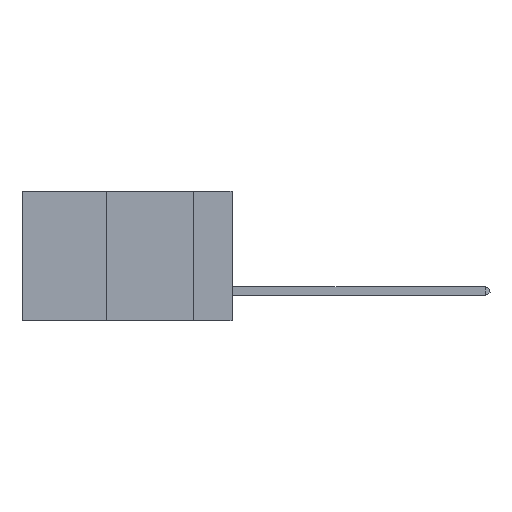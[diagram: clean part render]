
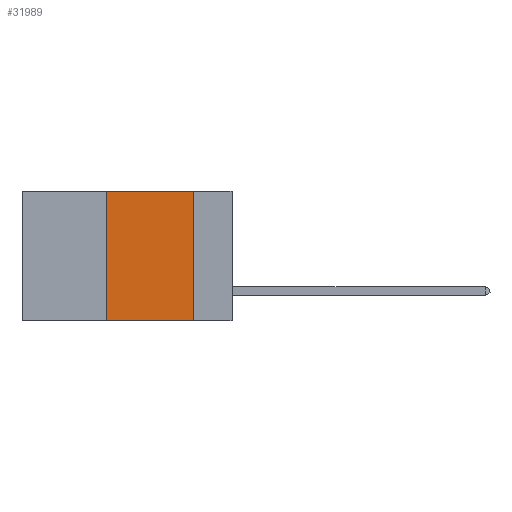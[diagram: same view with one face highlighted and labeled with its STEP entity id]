
A CAD part, left-side view. The second image highlights one B-rep face of the part: STEP entity #31989.
In plain terms, the highlighted planar face has unit normal (-1, 0, 0).
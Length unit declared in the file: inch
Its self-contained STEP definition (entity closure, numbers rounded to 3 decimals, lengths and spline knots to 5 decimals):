
#754 = CARTESIAN_POINT ( 'NONE',  ( 0., 0.11, 0. ) ) ;
#1330 = VERTEX_POINT ( 'NONE', #34725 ) ;
#3854 = CARTESIAN_POINT ( 'NONE',  ( 0., 0.36, 0. ) ) ;
#4259 = ORIENTED_EDGE ( 'NONE', *, *, #38365, .F. ) ;
#5767 = ORIENTED_EDGE ( 'NONE', *, *, #8758, .T. ) ;
#7262 = VECTOR ( 'NONE', #40436, 39.37008 ) ;
#8001 = VERTEX_POINT ( 'NONE', #3854 ) ;
#8758 = EDGE_CURVE ( 'NONE', #26494, #27726, #16987, .T. ) ;
#10231 = EDGE_CURVE ( 'NONE', #26494, #8001, #16358, .T. ) ;
#12664 = PLANE ( 'NONE',  #30285 ) ;
#12717 = VECTOR ( 'NONE', #30835, 39.37008 ) ;
#14123 = ORIENTED_EDGE ( 'NONE', *, *, #31626, .F. ) ;
#14644 = CARTESIAN_POINT ( 'NONE',  ( 0., 0.36, 0. ) ) ;
#14886 = EDGE_LOOP ( 'NONE', ( #14123, #4259, #38941, #5767 ) ) ;
#16358 = LINE ( 'NONE', #14644, #23242 ) ;
#16987 = LINE ( 'NONE', #34249, #12717 ) ;
#19331 = DIRECTION ( 'NONE',  ( 1., 0., 0. ) ) ;
#21008 = FACE_OUTER_BOUND ( 'NONE', #14886, .T. ) ;
#21571 = VECTOR ( 'NONE', #30937, 39.37008 ) ;
#23242 = VECTOR ( 'NONE', #28474, 39.37008 ) ;
#23522 = CARTESIAN_POINT ( 'NONE',  ( 0., 0.6, 0. ) ) ;
#25313 = LINE ( 'NONE', #23522, #7262 ) ;
#26494 = VERTEX_POINT ( 'NONE', #32504 ) ;
#27726 = VERTEX_POINT ( 'NONE', #35566 ) ;
#28474 = DIRECTION ( 'NONE',  ( 0., 0., 1. ) ) ;
#30285 = AXIS2_PLACEMENT_3D ( 'NONE', #36721, #19331, #43178 ) ;
#30835 = DIRECTION ( 'NONE',  ( 0., -1., 0. ) ) ;
#30937 = DIRECTION ( 'NONE',  ( 0., 0., -1. ) ) ;
#31626 = EDGE_CURVE ( 'NONE', #1330, #27726, #38563, .T. ) ;
#31989 = ADVANCED_FACE ( 'NONE', ( #21008 ), #12664, .F. ) ;
#32504 = CARTESIAN_POINT ( 'NONE',  ( 0., 0.36, -0.37 ) ) ;
#34249 = CARTESIAN_POINT ( 'NONE',  ( 0., 0.6, -0.37 ) ) ;
#34725 = CARTESIAN_POINT ( 'NONE',  ( 0., 0.11, 0. ) ) ;
#35566 = CARTESIAN_POINT ( 'NONE',  ( 0., 0.11, -0.37 ) ) ;
#36721 = CARTESIAN_POINT ( 'NONE',  ( 0., 0.6, 0. ) ) ;
#38365 = EDGE_CURVE ( 'NONE', #8001, #1330, #25313, .T. ) ;
#38563 = LINE ( 'NONE', #754, #21571 ) ;
#38941 = ORIENTED_EDGE ( 'NONE', *, *, #10231, .F. ) ;
#40436 = DIRECTION ( 'NONE',  ( 0., -1., 0. ) ) ;
#43178 = DIRECTION ( 'NONE',  ( 0., 0., -1. ) ) ;
